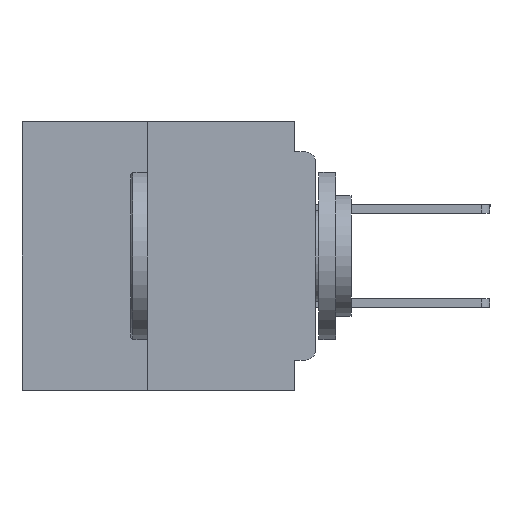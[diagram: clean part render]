
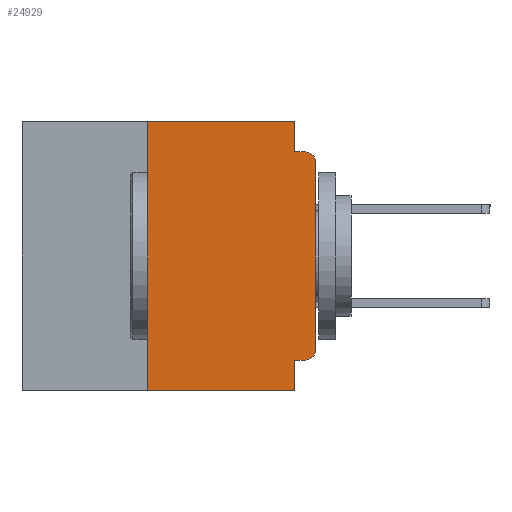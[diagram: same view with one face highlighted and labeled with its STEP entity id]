
A CAD part, left-side view. The second image highlights one B-rep face of the part: STEP entity #24929.
In plain terms, the highlighted planar face has unit normal (-1, 0, 0).
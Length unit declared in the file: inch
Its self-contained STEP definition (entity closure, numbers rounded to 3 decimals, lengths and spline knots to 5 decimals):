
#1254 = DIRECTION ( 'NONE',  ( 0., 0., 1. ) ) ;
#2586 = ORIENTED_EDGE ( 'NONE', *, *, #30137, .T. ) ;
#2599 = CARTESIAN_POINT ( 'NONE',  ( 0., 0.031, -0.4 ) ) ;
#2766 = EDGE_CURVE ( 'NONE', #39313, #15885, #11042, .T. ) ;
#2806 = ORIENTED_EDGE ( 'NONE', *, *, #36696, .F. ) ;
#3112 = ORIENTED_EDGE ( 'NONE', *, *, #8672, .F. ) ;
#3132 = PLANE ( 'NONE',  #6802 ) ;
#4687 = EDGE_CURVE ( 'NONE', #29308, #22912, #26803, .T. ) ;
#4891 = LINE ( 'NONE', #6191, #21219 ) ;
#5575 = VECTOR ( 'NONE', #12489, 39.37008 ) ;
#6191 = CARTESIAN_POINT ( 'NONE',  ( 0., 0.437, -0.4 ) ) ;
#6195 = CARTESIAN_POINT ( 'NONE',  ( 0., 0., -0.355 ) ) ;
#6802 = AXIS2_PLACEMENT_3D ( 'NONE', #29171, #39028, #19552 ) ;
#6992 = CARTESIAN_POINT ( 'NONE',  ( 0., 0.015, -0.06 ) ) ;
#7108 = EDGE_LOOP ( 'NONE', ( #23493, #10025, #3112, #2806, #20929, #14597, #2586, #19937, #26264, #21791 ) ) ;
#8672 = EDGE_CURVE ( 'NONE', #23783, #17381, #40268, .T. ) ;
#9043 = CARTESIAN_POINT ( 'NONE',  ( 0., 0.031, -0.4 ) ) ;
#9049 = VERTEX_POINT ( 'NONE', #28165 ) ;
#9345 = CARTESIAN_POINT ( 'NONE',  ( 0., 0., -0.34 ) ) ;
#9509 = DIRECTION ( 'NONE',  ( 0., -1., 0. ) ) ;
#9942 = VECTOR ( 'NONE', #10738, 39.37008 ) ;
#10025 = ORIENTED_EDGE ( 'NONE', *, *, #28953, .T. ) ;
#10312 = DIRECTION ( 'NONE',  ( 0., 0., -1. ) ) ;
#10738 = DIRECTION ( 'NONE',  ( 0., 0., 1. ) ) ;
#11042 = CIRCLE ( 'NONE', #35061, 0.015 ) ;
#12489 = DIRECTION ( 'NONE',  ( 0., 0., -1. ) ) ;
#13755 = FACE_OUTER_BOUND ( 'NONE', #7108, .T. ) ;
#13920 = CARTESIAN_POINT ( 'NONE',  ( 0., 0., 0. ) ) ;
#14329 = LINE ( 'NONE', #2599, #5575 ) ;
#14377 = VECTOR ( 'NONE', #16637, 39.37008 ) ;
#14597 = ORIENTED_EDGE ( 'NONE', *, *, #27310, .F. ) ;
#15885 = VERTEX_POINT ( 'NONE', #9345 ) ;
#16495 = CARTESIAN_POINT ( 'NONE',  ( 0., 0., -0.045 ) ) ;
#16637 = DIRECTION ( 'NONE',  ( 0., -1., 0. ) ) ;
#16825 = CARTESIAN_POINT ( 'NONE',  ( 0., 0.015, -0.045 ) ) ;
#17109 = LINE ( 'NONE', #23922, #22641 ) ;
#17381 = VERTEX_POINT ( 'NONE', #16825 ) ;
#18166 = AXIS2_PLACEMENT_3D ( 'NONE', #6992, #29753, #10312 ) ;
#19479 = CARTESIAN_POINT ( 'NONE',  ( 0., 0.015, -0.355 ) ) ;
#19552 = DIRECTION ( 'NONE',  ( 0., 0., -1. ) ) ;
#19937 = ORIENTED_EDGE ( 'NONE', *, *, #24215, .F. ) ;
#20412 = CARTESIAN_POINT ( 'NONE',  ( 0., 0.25, -0.4 ) ) ;
#20910 = LINE ( 'NONE', #6195, #27486 ) ;
#20929 = ORIENTED_EDGE ( 'NONE', *, *, #4687, .F. ) ;
#21219 = VECTOR ( 'NONE', #9509, 39.37008 ) ;
#21791 = ORIENTED_EDGE ( 'NONE', *, *, #2766, .T. ) ;
#22641 = VECTOR ( 'NONE', #1254, 39.37008 ) ;
#22912 = VERTEX_POINT ( 'NONE', #28583 ) ;
#23493 = ORIENTED_EDGE ( 'NONE', *, *, #31256, .T. ) ;
#23783 = VERTEX_POINT ( 'NONE', #36109 ) ;
#23922 = CARTESIAN_POINT ( 'NONE',  ( 0., 0.25, -0.4 ) ) ;
#24215 = EDGE_CURVE ( 'NONE', #29927, #41664, #14329, .T. ) ;
#24929 = ADVANCED_FACE ( 'NONE', ( #13755 ), #3132, .F. ) ;
#25710 = DIRECTION ( 'NONE',  ( 0., 1., 0. ) ) ;
#26264 = ORIENTED_EDGE ( 'NONE', *, *, #35874, .F. ) ;
#26803 = LINE ( 'NONE', #27289, #34435 ) ;
#27289 = CARTESIAN_POINT ( 'NONE',  ( 0., 0.437, 0. ) ) ;
#27310 = EDGE_CURVE ( 'NONE', #37582, #29308, #17109, .T. ) ;
#27486 = VECTOR ( 'NONE', #25710, 39.37008 ) ;
#28165 = CARTESIAN_POINT ( 'NONE',  ( 0., 0., -0.06 ) ) ;
#28213 = LINE ( 'NONE', #13920, #9942 ) ;
#28583 = CARTESIAN_POINT ( 'NONE',  ( 0., 0.031, 0. ) ) ;
#28953 = EDGE_CURVE ( 'NONE', #9049, #17381, #33233, .T. ) ;
#29171 = CARTESIAN_POINT ( 'NONE',  ( 0., 0.437, 0. ) ) ;
#29308 = VERTEX_POINT ( 'NONE', #34843 ) ;
#29477 = VECTOR ( 'NONE', #34957, 39.37008 ) ;
#29753 = DIRECTION ( 'NONE',  ( -1., 0., 0. ) ) ;
#29927 = VERTEX_POINT ( 'NONE', #37654 ) ;
#30137 = EDGE_CURVE ( 'NONE', #37582, #41664, #4891, .T. ) ;
#30485 = LINE ( 'NONE', #31684, #29477 ) ;
#30578 = DIRECTION ( 'NONE',  ( 0., -1., 0. ) ) ;
#31256 = EDGE_CURVE ( 'NONE', #15885, #9049, #28213, .T. ) ;
#31684 = CARTESIAN_POINT ( 'NONE',  ( 0., 0.031, 0. ) ) ;
#32888 = DIRECTION ( 'NONE',  ( 0., 0., -1. ) ) ;
#33233 = CIRCLE ( 'NONE', #18166, 0.015 ) ;
#33407 = DIRECTION ( 'NONE',  ( -1., 0., 0. ) ) ;
#33852 = CARTESIAN_POINT ( 'NONE',  ( 0., 0.015, -0.34 ) ) ;
#34435 = VECTOR ( 'NONE', #30578, 39.37008 ) ;
#34843 = CARTESIAN_POINT ( 'NONE',  ( 0., 0.25, 0. ) ) ;
#34957 = DIRECTION ( 'NONE',  ( 0., 0., -1. ) ) ;
#35061 = AXIS2_PLACEMENT_3D ( 'NONE', #33852, #33407, #32888 ) ;
#35874 = EDGE_CURVE ( 'NONE', #39313, #29927, #20910, .T. ) ;
#36109 = CARTESIAN_POINT ( 'NONE',  ( 0., 0.031, -0.045 ) ) ;
#36696 = EDGE_CURVE ( 'NONE', #22912, #23783, #30485, .T. ) ;
#37582 = VERTEX_POINT ( 'NONE', #20412 ) ;
#37654 = CARTESIAN_POINT ( 'NONE',  ( 0., 0.031, -0.355 ) ) ;
#39028 = DIRECTION ( 'NONE',  ( 1., 0., 0. ) ) ;
#39313 = VERTEX_POINT ( 'NONE', #19479 ) ;
#40268 = LINE ( 'NONE', #16495, #14377 ) ;
#41664 = VERTEX_POINT ( 'NONE', #9043 ) ;
